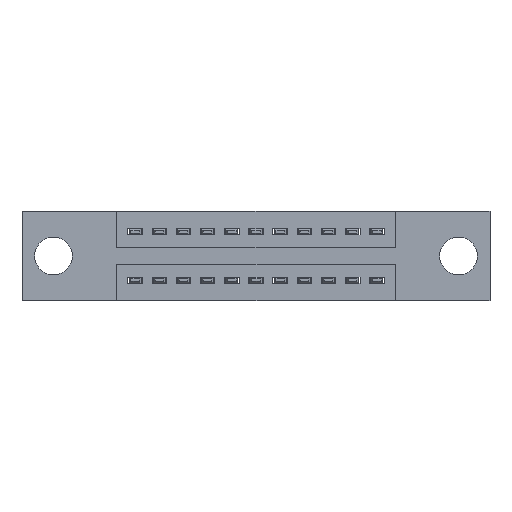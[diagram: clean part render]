
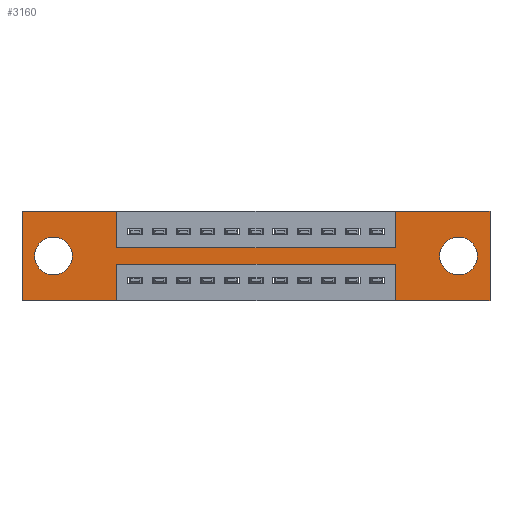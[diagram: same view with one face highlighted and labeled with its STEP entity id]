
A CAD part, front view. The second image highlights one B-rep face of the part: STEP entity #3160.
In plain terms, the highlighted planar face has unit normal (0, -1, 0).
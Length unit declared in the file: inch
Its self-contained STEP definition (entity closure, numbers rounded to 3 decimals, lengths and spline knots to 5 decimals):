
#3 = EDGE_LOOP ( 'NONE', ( #9990, #9393 ) ) ;
#75 = FACE_BOUND ( 'NONE', #3, .T. ) ;
#570 = VECTOR ( 'NONE', #3182, 39.37008 ) ;
#620 = CARTESIAN_POINT ( 'NONE',  ( 1.805, 0., -0.185 ) ) ;
#765 = VERTEX_POINT ( 'NONE', #4318 ) ;
#813 = DIRECTION ( 'NONE',  ( 0., 0., -1. ) ) ;
#874 = DIRECTION ( 'NONE',  ( 0., 0., 1. ) ) ;
#966 = LINE ( 'NONE', #6855, #5080 ) ;
#1025 = LINE ( 'NONE', #2149, #8741 ) ;
#1039 = CARTESIAN_POINT ( 'NONE',  ( 0., 0., -0.37 ) ) ;
#1306 = CARTESIAN_POINT ( 'NONE',  ( 0., 0., -0.37 ) ) ;
#1495 = ORIENTED_EDGE ( 'NONE', *, *, #7465, .F. ) ;
#1571 = EDGE_CURVE ( 'NONE', #7078, #2028, #11461, .T. ) ;
#1593 = ORIENTED_EDGE ( 'NONE', *, *, #10590, .F. ) ;
#1605 = DIRECTION ( 'NONE',  ( -1., 0., 0. ) ) ;
#1616 = CARTESIAN_POINT ( 'NONE',  ( 0.13, 0., -0.107 ) ) ;
#1784 = CARTESIAN_POINT ( 'NONE',  ( 0.3925, 0., 0. ) ) ;
#2011 = EDGE_CURVE ( 'NONE', #5858, #7087, #12824, .T. ) ;
#2028 = VERTEX_POINT ( 'NONE', #4813 ) ;
#2058 = CARTESIAN_POINT ( 'NONE',  ( 0., 0., 0. ) ) ;
#2132 = EDGE_CURVE ( 'NONE', #7770, #7502, #9776, .T. ) ;
#2136 = FACE_OUTER_BOUND ( 'NONE', #3107, .T. ) ;
#2149 = CARTESIAN_POINT ( 'NONE',  ( 0., 0., 0. ) ) ;
#2152 = VERTEX_POINT ( 'NONE', #1039 ) ;
#2267 = VECTOR ( 'NONE', #10754, 39.37008 ) ;
#2533 = ORIENTED_EDGE ( 'NONE', *, *, #12128, .F. ) ;
#2562 = EDGE_CURVE ( 'NONE', #6123, #2745, #7916, .T. ) ;
#2574 = ORIENTED_EDGE ( 'NONE', *, *, #9307, .F. ) ;
#2606 = EDGE_CURVE ( 'NONE', #11725, #7770, #3013, .T. ) ;
#2609 = VECTOR ( 'NONE', #11929, 39.37008 ) ;
#2696 = LINE ( 'NONE', #1784, #10810 ) ;
#2702 = CARTESIAN_POINT ( 'NONE',  ( 1.935, 0., 0. ) ) ;
#2737 = EDGE_CURVE ( 'NONE', #5836, #765, #1025, .T. ) ;
#2745 = VERTEX_POINT ( 'NONE', #11986 ) ;
#2869 = DIRECTION ( 'NONE',  ( 0., 1., 0. ) ) ;
#2933 = EDGE_CURVE ( 'NONE', #7087, #5858, #4078, .T. ) ;
#2997 = PLANE ( 'NONE',  #5076 ) ;
#3013 = LINE ( 'NONE', #7162, #3028 ) ;
#3028 = VECTOR ( 'NONE', #10068, 39.37008 ) ;
#3052 = CARTESIAN_POINT ( 'NONE',  ( 1.805, 0., -0.263 ) ) ;
#3107 = EDGE_LOOP ( 'NONE', ( #2574, #13009, #3643, #7148, #11350, #4901, #9316, #1495, #7790, #12549, #1593, #2533 ) ) ;
#3160 = ADVANCED_FACE ( 'NONE', ( #75, #8154, #2136 ), #2997, .T. ) ;
#3182 = DIRECTION ( 'NONE',  ( -1., 0., 0. ) ) ;
#3290 = VERTEX_POINT ( 'NONE', #12624 ) ;
#3542 = ORIENTED_EDGE ( 'NONE', *, *, #1571, .T. ) ;
#3560 = LINE ( 'NONE', #1306, #4907 ) ;
#3633 = CARTESIAN_POINT ( 'NONE',  ( 0.3925, 0., -0.22 ) ) ;
#3643 = ORIENTED_EDGE ( 'NONE', *, *, #2562, .F. ) ;
#3861 = LINE ( 'NONE', #6768, #7758 ) ;
#3906 = CARTESIAN_POINT ( 'NONE',  ( 0.13, 0., -0.185 ) ) ;
#4078 = CIRCLE ( 'NONE', #11456, 0.078 ) ;
#4218 = EDGE_LOOP ( 'NONE', ( #3542, #6501 ) ) ;
#4273 = EDGE_CURVE ( 'NONE', #8226, #11725, #3861, .T. ) ;
#4318 = CARTESIAN_POINT ( 'NONE',  ( 0.3925, 0., 0. ) ) ;
#4444 = EDGE_CURVE ( 'NONE', #2745, #12518, #6213, .T. ) ;
#4755 = CARTESIAN_POINT ( 'NONE',  ( 1.5425, 0., -0.37 ) ) ;
#4813 = CARTESIAN_POINT ( 'NONE',  ( 0.13, 0., -0.263 ) ) ;
#4901 = ORIENTED_EDGE ( 'NONE', *, *, #2606, .F. ) ;
#4907 = VECTOR ( 'NONE', #7591, 39.37008 ) ;
#4919 = CIRCLE ( 'NONE', #11675, 0.078 ) ;
#5014 = AXIS2_PLACEMENT_3D ( 'NONE', #10885, #9960, #7859 ) ;
#5076 = AXIS2_PLACEMENT_3D ( 'NONE', #12160, #6155, #6270 ) ;
#5080 = VECTOR ( 'NONE', #10881, 39.37008 ) ;
#5384 = DIRECTION ( 'NONE',  ( 0., 0., 1. ) ) ;
#5552 = DIRECTION ( 'NONE',  ( 1., 0., 0. ) ) ;
#5671 = DIRECTION ( 'NONE',  ( 0., 0., -1. ) ) ;
#5686 = LINE ( 'NONE', #8662, #11596 ) ;
#5764 = VECTOR ( 'NONE', #5894, 39.37008 ) ;
#5836 = VERTEX_POINT ( 'NONE', #2058 ) ;
#5858 = VERTEX_POINT ( 'NONE', #12146 ) ;
#5894 = DIRECTION ( 'NONE',  ( 0., 0., 1. ) ) ;
#6011 = DIRECTION ( 'NONE',  ( 0., 1., 0. ) ) ;
#6123 = VERTEX_POINT ( 'NONE', #4755 ) ;
#6155 = DIRECTION ( 'NONE',  ( 0., -1., 0. ) ) ;
#6213 = LINE ( 'NONE', #9145, #570 ) ;
#6270 = DIRECTION ( 'NONE',  ( 0., 0., -1. ) ) ;
#6501 = ORIENTED_EDGE ( 'NONE', *, *, #11127, .T. ) ;
#6558 = CARTESIAN_POINT ( 'NONE',  ( 1.5425, 0., 0. ) ) ;
#6768 = CARTESIAN_POINT ( 'NONE',  ( 1.5425, 0., 0. ) ) ;
#6855 = CARTESIAN_POINT ( 'NONE',  ( 0.3925, 0., -0.37 ) ) ;
#7026 = AXIS2_PLACEMENT_3D ( 'NONE', #3906, #6011, #9054 ) ;
#7078 = VERTEX_POINT ( 'NONE', #1616 ) ;
#7087 = VERTEX_POINT ( 'NONE', #3052 ) ;
#7148 = ORIENTED_EDGE ( 'NONE', *, *, #10761, .F. ) ;
#7162 = CARTESIAN_POINT ( 'NONE',  ( 0., 0., 0. ) ) ;
#7370 = DIRECTION ( 'NONE',  ( 0., 1., 0. ) ) ;
#7465 = EDGE_CURVE ( 'NONE', #3290, #8226, #5686, .T. ) ;
#7502 = VERTEX_POINT ( 'NONE', #10762 ) ;
#7577 = CARTESIAN_POINT ( 'NONE',  ( 0.13, 0., -0.185 ) ) ;
#7591 = DIRECTION ( 'NONE',  ( -1., 0., 0. ) ) ;
#7720 = CARTESIAN_POINT ( 'NONE',  ( 1.5425, 0., -0.37 ) ) ;
#7758 = VECTOR ( 'NONE', #874, 39.37008 ) ;
#7770 = VERTEX_POINT ( 'NONE', #11406 ) ;
#7790 = ORIENTED_EDGE ( 'NONE', *, *, #10802, .F. ) ;
#7859 = DIRECTION ( 'NONE',  ( 0., 0., -1. ) ) ;
#7916 = LINE ( 'NONE', #7720, #2609 ) ;
#8014 = CARTESIAN_POINT ( 'NONE',  ( 0., 0., 0. ) ) ;
#8078 = LINE ( 'NONE', #8014, #5764 ) ;
#8120 = VECTOR ( 'NONE', #1605, 39.37008 ) ;
#8154 = FACE_BOUND ( 'NONE', #4218, .T. ) ;
#8226 = VERTEX_POINT ( 'NONE', #9217 ) ;
#8662 = CARTESIAN_POINT ( 'NONE',  ( 0.3925, 0., -0.15 ) ) ;
#8741 = VECTOR ( 'NONE', #12239, 39.37008 ) ;
#9054 = DIRECTION ( 'NONE',  ( 0., 0., 1. ) ) ;
#9145 = CARTESIAN_POINT ( 'NONE',  ( 0.3925, 0., -0.22 ) ) ;
#9217 = CARTESIAN_POINT ( 'NONE',  ( 1.5425, 0., -0.15 ) ) ;
#9307 = EDGE_CURVE ( 'NONE', #12518, #12148, #966, .T. ) ;
#9316 = ORIENTED_EDGE ( 'NONE', *, *, #4273, .F. ) ;
#9393 = ORIENTED_EDGE ( 'NONE', *, *, #2933, .T. ) ;
#9656 = CARTESIAN_POINT ( 'NONE',  ( 0.3925, 0., -0.37 ) ) ;
#9776 = LINE ( 'NONE', #2702, #2267 ) ;
#9960 = DIRECTION ( 'NONE',  ( 0., 1., 0. ) ) ;
#9990 = ORIENTED_EDGE ( 'NONE', *, *, #2011, .T. ) ;
#10068 = DIRECTION ( 'NONE',  ( 1., 0., 0. ) ) ;
#10590 = EDGE_CURVE ( 'NONE', #2152, #5836, #8078, .T. ) ;
#10754 = DIRECTION ( 'NONE',  ( 0., 0., -1. ) ) ;
#10761 = EDGE_CURVE ( 'NONE', #7502, #6123, #3560, .T. ) ;
#10762 = CARTESIAN_POINT ( 'NONE',  ( 1.935, 0., -0.37 ) ) ;
#10802 = EDGE_CURVE ( 'NONE', #765, #3290, #2696, .T. ) ;
#10810 = VECTOR ( 'NONE', #5671, 39.37008 ) ;
#10881 = DIRECTION ( 'NONE',  ( 0., 0., -1. ) ) ;
#10885 = CARTESIAN_POINT ( 'NONE',  ( 1.805, 0., -0.185 ) ) ;
#11127 = EDGE_CURVE ( 'NONE', #2028, #7078, #4919, .T. ) ;
#11350 = ORIENTED_EDGE ( 'NONE', *, *, #2132, .F. ) ;
#11406 = CARTESIAN_POINT ( 'NONE',  ( 1.935, 0., 0. ) ) ;
#11456 = AXIS2_PLACEMENT_3D ( 'NONE', #620, #2869, #813 ) ;
#11461 = CIRCLE ( 'NONE', #7026, 0.078 ) ;
#11568 = LINE ( 'NONE', #11635, #8120 ) ;
#11596 = VECTOR ( 'NONE', #5552, 39.37008 ) ;
#11635 = CARTESIAN_POINT ( 'NONE',  ( 0., 0., -0.37 ) ) ;
#11675 = AXIS2_PLACEMENT_3D ( 'NONE', #7577, #7370, #5384 ) ;
#11725 = VERTEX_POINT ( 'NONE', #6558 ) ;
#11929 = DIRECTION ( 'NONE',  ( 0., 0., 1. ) ) ;
#11986 = CARTESIAN_POINT ( 'NONE',  ( 1.5425, 0., -0.22 ) ) ;
#12128 = EDGE_CURVE ( 'NONE', #12148, #2152, #11568, .T. ) ;
#12146 = CARTESIAN_POINT ( 'NONE',  ( 1.805, 0., -0.107 ) ) ;
#12148 = VERTEX_POINT ( 'NONE', #9656 ) ;
#12160 = CARTESIAN_POINT ( 'NONE',  ( 0., 0., -0.37 ) ) ;
#12239 = DIRECTION ( 'NONE',  ( 1., 0., 0. ) ) ;
#12518 = VERTEX_POINT ( 'NONE', #3633 ) ;
#12549 = ORIENTED_EDGE ( 'NONE', *, *, #2737, .F. ) ;
#12624 = CARTESIAN_POINT ( 'NONE',  ( 0.3925, 0., -0.15 ) ) ;
#12824 = CIRCLE ( 'NONE', #5014, 0.078 ) ;
#13009 = ORIENTED_EDGE ( 'NONE', *, *, #4444, .F. ) ;
